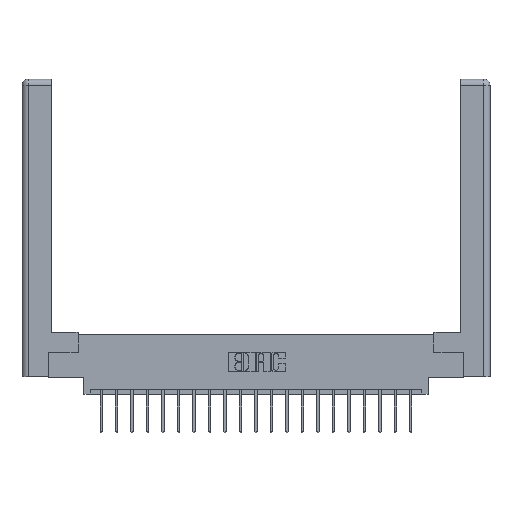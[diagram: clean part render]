
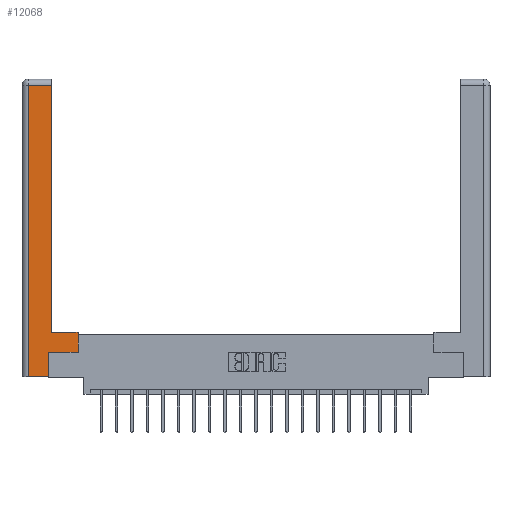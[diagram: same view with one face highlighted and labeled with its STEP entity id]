
A CAD part, top view. The second image highlights one B-rep face of the part: STEP entity #12068.
In plain terms, the highlighted planar face has unit normal (0, 0, 1).
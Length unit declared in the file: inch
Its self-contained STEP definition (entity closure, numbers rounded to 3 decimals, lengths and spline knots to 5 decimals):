
#122 = DIRECTION ( 'NONE',  ( -1., 0., 0. ) ) ;
#263 = VECTOR ( 'NONE', #962, 39.37008 ) ;
#623 = VERTEX_POINT ( 'NONE', #11714 ) ;
#649 = ORIENTED_EDGE ( 'NONE', *, *, #11842, .T. ) ;
#650 = DIRECTION ( 'NONE',  ( 0., -1., 0. ) ) ;
#962 = DIRECTION ( 'NONE',  ( 0., 1., 0. ) ) ;
#1082 = VECTOR ( 'NONE', #2830, 39.37008 ) ;
#1149 = EDGE_CURVE ( 'NONE', #623, #15968, #18195, .T. ) ;
#1187 = CARTESIAN_POINT ( 'NONE',  ( 0.565, 0.245, 0. ) ) ;
#2559 = VECTOR ( 'NONE', #122, 39.37008 ) ;
#2830 = DIRECTION ( 'NONE',  ( 0., 1., 0. ) ) ;
#2839 = LINE ( 'NONE', #3979, #8651 ) ;
#3182 = CARTESIAN_POINT ( 'NONE',  ( 0.265, 0., 0. ) ) ;
#3979 = CARTESIAN_POINT ( 'NONE',  ( 0.0615, 0., 0. ) ) ;
#4372 = VERTEX_POINT ( 'NONE', #17831 ) ;
#4419 = VECTOR ( 'NONE', #5867, 39.37008 ) ;
#4723 = EDGE_CURVE ( 'NONE', #13170, #19033, #2839, .T. ) ;
#4771 = VECTOR ( 'NONE', #13892, 39.37008 ) ;
#5059 = LINE ( 'NONE', #19692, #263 ) ;
#5119 = DIRECTION ( 'NONE',  ( 1., 0., 0. ) ) ;
#5153 = PLANE ( 'NONE',  #8257 ) ;
#5330 = EDGE_CURVE ( 'NONE', #19033, #7207, #6535, .T. ) ;
#5695 = CARTESIAN_POINT ( 'NONE',  ( 0.265, 0.245, 0. ) ) ;
#5867 = DIRECTION ( 'NONE',  ( -1., 0., 0. ) ) ;
#6535 = LINE ( 'NONE', #3182, #19363 ) ;
#6575 = DIRECTION ( 'NONE',  ( 0., 0., -1. ) ) ;
#6881 = CARTESIAN_POINT ( 'NONE',  ( 0.295, 0.45, 0. ) ) ;
#7127 = FACE_OUTER_BOUND ( 'NONE', #15337, .T. ) ;
#7181 = VERTEX_POINT ( 'NONE', #18831 ) ;
#7207 = VERTEX_POINT ( 'NONE', #20563 ) ;
#7314 = LINE ( 'NONE', #6881, #2559 ) ;
#7734 = ORIENTED_EDGE ( 'NONE', *, *, #5330, .T. ) ;
#8185 = EDGE_CURVE ( 'NONE', #19583, #623, #18706, .T. ) ;
#8257 = AXIS2_PLACEMENT_3D ( 'NONE', #11815, #6575, #8403 ) ;
#8271 = EDGE_CURVE ( 'NONE', #7181, #4372, #5059, .T. ) ;
#8403 = DIRECTION ( 'NONE',  ( -1., 0., 0. ) ) ;
#8651 = VECTOR ( 'NONE', #650, 39.37008 ) ;
#9346 = ORIENTED_EDGE ( 'NONE', *, *, #18989, .T. ) ;
#11591 = VECTOR ( 'NONE', #12729, 39.37008 ) ;
#11714 = CARTESIAN_POINT ( 'NONE',  ( 0.565, 0.245, 0. ) ) ;
#11815 = CARTESIAN_POINT ( 'NONE',  ( 0., 0., 0. ) ) ;
#11842 = EDGE_CURVE ( 'NONE', #7207, #19583, #14742, .T. ) ;
#12068 = ADVANCED_FACE ( 'NONE', ( #7127 ), #5153, .F. ) ;
#12335 = ORIENTED_EDGE ( 'NONE', *, *, #4723, .T. ) ;
#12414 = CARTESIAN_POINT ( 'NONE',  ( 0.0615, 0., 0. ) ) ;
#12729 = DIRECTION ( 'NONE',  ( 1., 0., 0. ) ) ;
#12756 = CARTESIAN_POINT ( 'NONE',  ( 0.565, 0.45, 0. ) ) ;
#12822 = LINE ( 'NONE', #14215, #4419 ) ;
#13036 = ORIENTED_EDGE ( 'NONE', *, *, #18023, .T. ) ;
#13170 = VERTEX_POINT ( 'NONE', #14158 ) ;
#13892 = DIRECTION ( 'NONE',  ( 0., 1., 0. ) ) ;
#14158 = CARTESIAN_POINT ( 'NONE',  ( 0.0615, 2.94, 0. ) ) ;
#14215 = CARTESIAN_POINT ( 'NONE',  ( 0.0615, 2.94, 0. ) ) ;
#14742 = LINE ( 'NONE', #5695, #4771 ) ;
#15337 = EDGE_LOOP ( 'NONE', ( #19395, #13036, #12335, #7734, #649, #18124, #15613, #9346 ) ) ;
#15613 = ORIENTED_EDGE ( 'NONE', *, *, #1149, .T. ) ;
#15968 = VERTEX_POINT ( 'NONE', #12756 ) ;
#16508 = CARTESIAN_POINT ( 'NONE',  ( 0.565, 0.45, 0. ) ) ;
#17831 = CARTESIAN_POINT ( 'NONE',  ( 0.295, 2.94, 0. ) ) ;
#18023 = EDGE_CURVE ( 'NONE', #4372, #13170, #12822, .T. ) ;
#18124 = ORIENTED_EDGE ( 'NONE', *, *, #8185, .T. ) ;
#18195 = LINE ( 'NONE', #16508, #1082 ) ;
#18706 = LINE ( 'NONE', #1187, #11591 ) ;
#18831 = CARTESIAN_POINT ( 'NONE',  ( 0.295, 0.45, 0. ) ) ;
#18989 = EDGE_CURVE ( 'NONE', #15968, #7181, #7314, .T. ) ;
#19033 = VERTEX_POINT ( 'NONE', #12414 ) ;
#19363 = VECTOR ( 'NONE', #5119, 39.37008 ) ;
#19395 = ORIENTED_EDGE ( 'NONE', *, *, #8271, .T. ) ;
#19583 = VERTEX_POINT ( 'NONE', #20597 ) ;
#19692 = CARTESIAN_POINT ( 'NONE',  ( 0.295, 3., 0. ) ) ;
#20563 = CARTESIAN_POINT ( 'NONE',  ( 0.265, 0., 0. ) ) ;
#20597 = CARTESIAN_POINT ( 'NONE',  ( 0.265, 0.245, 0. ) ) ;
